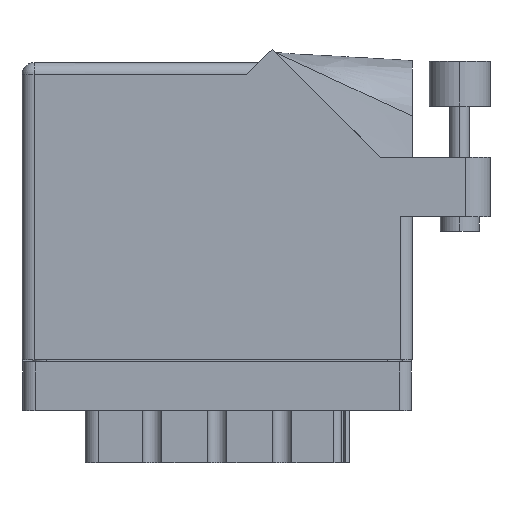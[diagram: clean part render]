
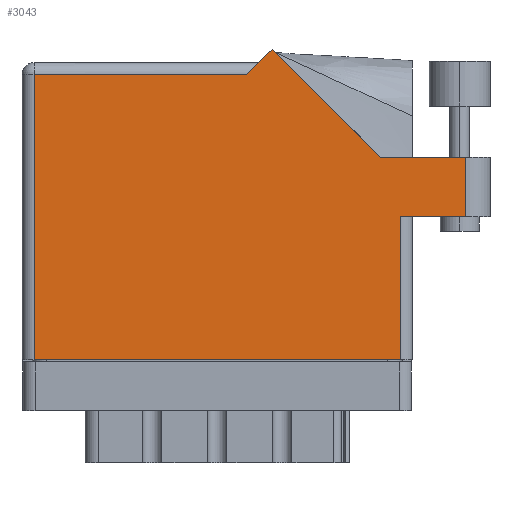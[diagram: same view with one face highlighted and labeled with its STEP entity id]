
A CAD part, front view. The second image highlights one B-rep face of the part: STEP entity #3043.
In plain terms, the highlighted face is planar.
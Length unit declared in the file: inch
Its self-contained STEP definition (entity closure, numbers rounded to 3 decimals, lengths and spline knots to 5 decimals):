
#376 = DIRECTION ( 'NONE',  ( 0., 0., -1. ) ) ;
#1304 = VERTEX_POINT ( 'NONE', #26712 ) ;
#1702 = AXIS2_PLACEMENT_3D ( 'NONE', #32193, #376, #32317 ) ;
#2165 = VERTEX_POINT ( 'NONE', #11304 ) ;
#2515 = ORIENTED_EDGE ( 'NONE', *, *, #33591, .T. ) ;
#3043 = ADVANCED_FACE ( 'NONE', ( #34517 ), #28907, .F. ) ;
#5514 = CARTESIAN_POINT ( 'NONE',  ( 2.01, 0.737, 0. ) ) ;
#5523 = VERTEX_POINT ( 'NONE', #31957 ) ;
#5986 = DIRECTION ( 'NONE',  ( -1., 0., 0. ) ) ;
#6130 = CARTESIAN_POINT ( 'NONE',  ( 0., 0., 0. ) ) ;
#6163 = EDGE_LOOP ( 'NONE', ( #7393, #28732, #24922, #15031, #13352, #2515, #28839, #8343, #27868 ) ) ;
#6374 = DIRECTION ( 'NONE',  ( 1., 0., 0. ) ) ;
#7320 = CARTESIAN_POINT ( 'NONE',  ( 1.155, 1.468, 0. ) ) ;
#7393 = ORIENTED_EDGE ( 'NONE', *, *, #16023, .T. ) ;
#7790 = CARTESIAN_POINT ( 'NONE',  ( 2.285, 1.044, 0. ) ) ;
#8036 = CARTESIAN_POINT ( 'NONE',  ( 1.84442, 1.044, 0. ) ) ;
#8216 = LINE ( 'NONE', #18836, #34317 ) ;
#8343 = ORIENTED_EDGE ( 'NONE', *, *, #13264, .T. ) ;
#8586 = VERTEX_POINT ( 'NONE', #34304 ) ;
#9673 = CARTESIAN_POINT ( 'NONE',  ( 1.948, 0.737, 0. ) ) ;
#10102 = LINE ( 'NONE', #5514, #19979 ) ;
#10781 = LINE ( 'NONE', #33222, #24754 ) ;
#11304 = CARTESIAN_POINT ( 'NONE',  ( 2.285, 0.737, 0. ) ) ;
#12502 = VECTOR ( 'NONE', #6374, 39.37008 ) ;
#13264 = EDGE_CURVE ( 'NONE', #16017, #5523, #16560, .T. ) ;
#13294 = VECTOR ( 'NONE', #22848, 39.37008 ) ;
#13300 = LINE ( 'NONE', #7790, #23240 ) ;
#13352 = ORIENTED_EDGE ( 'NONE', *, *, #22260, .T. ) ;
#13746 = LINE ( 'NONE', #34569, #13294 ) ;
#14387 = VERTEX_POINT ( 'NONE', #19660 ) ;
#14616 = EDGE_CURVE ( 'NONE', #28428, #28433, #13746, .T. ) ;
#15031 = ORIENTED_EDGE ( 'NONE', *, *, #14616, .T. ) ;
#15396 = EDGE_CURVE ( 'NONE', #2165, #14387, #13300, .T. ) ;
#15730 = DIRECTION ( 'NONE',  ( 0., -1., 0. ) ) ;
#16017 = VERTEX_POINT ( 'NONE', #31343 ) ;
#16023 = EDGE_CURVE ( 'NONE', #1304, #2165, #10102, .T. ) ;
#16560 = LINE ( 'NONE', #6130, #12502 ) ;
#16712 = EDGE_CURVE ( 'NONE', #14387, #28428, #36557, .T. ) ;
#17605 = VECTOR ( 'NONE', #32919, 39.37008 ) ;
#17868 = EDGE_CURVE ( 'NONE', #5523, #1304, #27915, .T. ) ;
#18459 = LINE ( 'NONE', #18543, #17605 ) ;
#18543 = CARTESIAN_POINT ( 'NONE',  ( 0., 1.468, 0. ) ) ;
#18836 = CARTESIAN_POINT ( 'NONE',  ( 0.062, 0., 0. ) ) ;
#18978 = VECTOR ( 'NONE', #5986, 39.37008 ) ;
#19660 = CARTESIAN_POINT ( 'NONE',  ( 2.285, 1.044, 0. ) ) ;
#19866 = DIRECTION ( 'NONE',  ( 1., 0., 0. ) ) ;
#19979 = VECTOR ( 'NONE', #19866, 39.37008 ) ;
#22260 = EDGE_CURVE ( 'NONE', #28433, #36085, #10781, .T. ) ;
#22848 = DIRECTION ( 'NONE',  ( -0.707, 0.707, 0. ) ) ;
#23240 = VECTOR ( 'NONE', #27971, 39.37008 ) ;
#23302 = CARTESIAN_POINT ( 'NONE',  ( 2.41, 1.044, 0. ) ) ;
#24754 = VECTOR ( 'NONE', #30180, 39.37008 ) ;
#24922 = ORIENTED_EDGE ( 'NONE', *, *, #16712, .T. ) ;
#25663 = VECTOR ( 'NONE', #35246, 39.37008 ) ;
#26712 = CARTESIAN_POINT ( 'NONE',  ( 1.948, 0.737, 0. ) ) ;
#26730 = EDGE_CURVE ( 'NONE', #8586, #16017, #8216, .T. ) ;
#27868 = ORIENTED_EDGE ( 'NONE', *, *, #17868, .T. ) ;
#27915 = LINE ( 'NONE', #9673, #25663 ) ;
#27971 = DIRECTION ( 'NONE',  ( 0., 1., 0. ) ) ;
#28428 = VERTEX_POINT ( 'NONE', #8036 ) ;
#28433 = VERTEX_POINT ( 'NONE', #36662 ) ;
#28732 = ORIENTED_EDGE ( 'NONE', *, *, #15396, .T. ) ;
#28839 = ORIENTED_EDGE ( 'NONE', *, *, #26730, .T. ) ;
#28907 = PLANE ( 'NONE',  #1702 ) ;
#30180 = DIRECTION ( 'NONE',  ( -0.707, -0.707, 0. ) ) ;
#31343 = CARTESIAN_POINT ( 'NONE',  ( 0.062, 0., 0. ) ) ;
#31957 = CARTESIAN_POINT ( 'NONE',  ( 1.948, 0., 0. ) ) ;
#32193 = CARTESIAN_POINT ( 'NONE',  ( 0., 1.53, 0. ) ) ;
#32317 = DIRECTION ( 'NONE',  ( -1., 0., 0. ) ) ;
#32919 = DIRECTION ( 'NONE',  ( -1., 0., 0. ) ) ;
#33222 = CARTESIAN_POINT ( 'NONE',  ( 1.217, 1.53, 0. ) ) ;
#33591 = EDGE_CURVE ( 'NONE', #36085, #8586, #18459, .T. ) ;
#34304 = CARTESIAN_POINT ( 'NONE',  ( 0.062, 1.468, 0. ) ) ;
#34317 = VECTOR ( 'NONE', #15730, 39.37008 ) ;
#34517 = FACE_OUTER_BOUND ( 'NONE', #6163, .T. ) ;
#34569 = CARTESIAN_POINT ( 'NONE',  ( 1.84442, 1.044, 0. ) ) ;
#35246 = DIRECTION ( 'NONE',  ( 0., 1., 0. ) ) ;
#36085 = VERTEX_POINT ( 'NONE', #7320 ) ;
#36557 = LINE ( 'NONE', #23302, #18978 ) ;
#36662 = CARTESIAN_POINT ( 'NONE',  ( 1.28771, 1.60071, 0. ) ) ;
